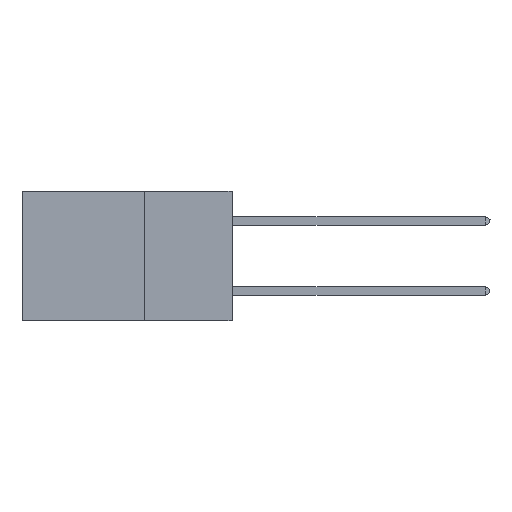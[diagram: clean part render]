
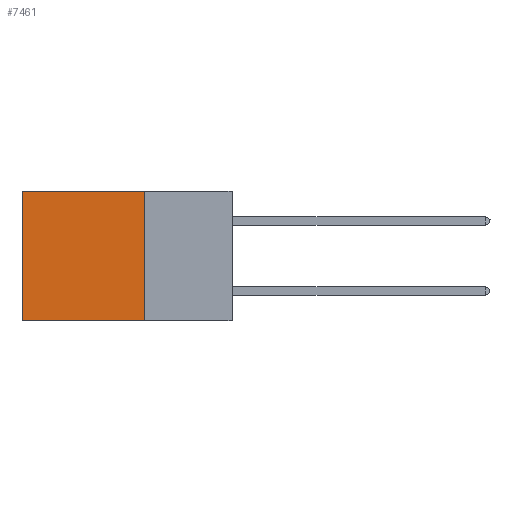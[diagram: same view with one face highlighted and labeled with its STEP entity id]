
A CAD part, left-side view. The second image highlights one B-rep face of the part: STEP entity #7461.
In plain terms, the highlighted planar face has unit normal (-1, 0, 0).
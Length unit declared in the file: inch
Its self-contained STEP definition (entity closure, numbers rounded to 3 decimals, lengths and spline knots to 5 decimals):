
#676 = DIRECTION ( 'NONE',  ( 0., 1., 0. ) ) ;
#3693 = VECTOR ( 'NONE', #18105, 39.37008 ) ;
#3829 = VERTEX_POINT ( 'NONE', #28569 ) ;
#5181 = AXIS2_PLACEMENT_3D ( 'NONE', #32557, #17601, #35257 ) ;
#6436 = LINE ( 'NONE', #24530, #30465 ) ;
#6903 = EDGE_LOOP ( 'NONE', ( #17093, #36971, #20717, #8722 ) ) ;
#7461 = ADVANCED_FACE ( 'NONE', ( #21049 ), #18351, .F. ) ;
#8722 = ORIENTED_EDGE ( 'NONE', *, *, #12813, .T. ) ;
#11765 = VECTOR ( 'NONE', #16662, 39.37008 ) ;
#12813 = EDGE_CURVE ( 'NONE', #3829, #32487, #6436, .T. ) ;
#13502 = CARTESIAN_POINT ( 'NONE',  ( 0.2875, 0.25, -0.37 ) ) ;
#15039 = CARTESIAN_POINT ( 'NONE',  ( 0.2875, 0.6, 0. ) ) ;
#16289 = CARTESIAN_POINT ( 'NONE',  ( 0.2875, 0.25, 0. ) ) ;
#16662 = DIRECTION ( 'NONE',  ( 0., 0., -1. ) ) ;
#17093 = ORIENTED_EDGE ( 'NONE', *, *, #33197, .T. ) ;
#17601 = DIRECTION ( 'NONE',  ( 1., 0., 0. ) ) ;
#18105 = DIRECTION ( 'NONE',  ( 0., 0., -1. ) ) ;
#18351 = PLANE ( 'NONE',  #5181 ) ;
#19049 = EDGE_CURVE ( 'NONE', #3829, #22239, #19762, .T. ) ;
#19762 = LINE ( 'NONE', #16289, #11765 ) ;
#20717 = ORIENTED_EDGE ( 'NONE', *, *, #19049, .F. ) ;
#21049 = FACE_OUTER_BOUND ( 'NONE', #6903, .T. ) ;
#22239 = VERTEX_POINT ( 'NONE', #25229 ) ;
#24249 = LINE ( 'NONE', #15039, #3693 ) ;
#24382 = CARTESIAN_POINT ( 'NONE',  ( 0.2875, 0.6, 0. ) ) ;
#24530 = CARTESIAN_POINT ( 'NONE',  ( 0.2875, 0.25, 0. ) ) ;
#25229 = CARTESIAN_POINT ( 'NONE',  ( 0.2875, 0.25, -0.37 ) ) ;
#25418 = LINE ( 'NONE', #13502, #35972 ) ;
#26783 = EDGE_CURVE ( 'NONE', #22239, #35831, #25418, .T. ) ;
#28569 = CARTESIAN_POINT ( 'NONE',  ( 0.2875, 0.25, 0. ) ) ;
#30465 = VECTOR ( 'NONE', #676, 39.37008 ) ;
#31164 = DIRECTION ( 'NONE',  ( 0., 1., 0. ) ) ;
#32487 = VERTEX_POINT ( 'NONE', #24382 ) ;
#32557 = CARTESIAN_POINT ( 'NONE',  ( 0.2875, 0.25, 0. ) ) ;
#33197 = EDGE_CURVE ( 'NONE', #32487, #35831, #24249, .T. ) ;
#35257 = DIRECTION ( 'NONE',  ( 0., 0., -1. ) ) ;
#35823 = CARTESIAN_POINT ( 'NONE',  ( 0.2875, 0.6, -0.37 ) ) ;
#35831 = VERTEX_POINT ( 'NONE', #35823 ) ;
#35972 = VECTOR ( 'NONE', #31164, 39.37008 ) ;
#36971 = ORIENTED_EDGE ( 'NONE', *, *, #26783, .F. ) ;
